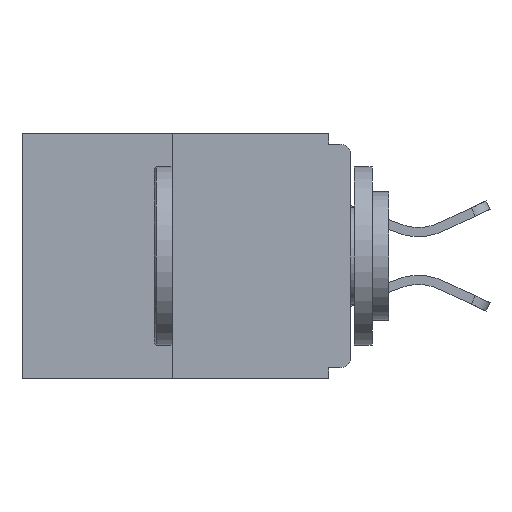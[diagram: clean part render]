
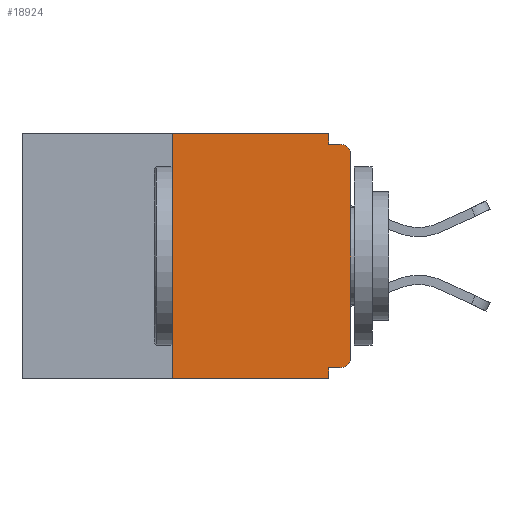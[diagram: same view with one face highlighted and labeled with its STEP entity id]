
A CAD part, left-side view. The second image highlights one B-rep face of the part: STEP entity #18924.
In plain terms, the highlighted planar face has unit normal (-1, 0, 0).
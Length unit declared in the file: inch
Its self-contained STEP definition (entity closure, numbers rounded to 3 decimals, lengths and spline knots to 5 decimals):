
#227 = EDGE_LOOP ( 'NONE', ( #14195, #5316, #4825, #1654, #13470, #17255, #25778, #17667, #17939, #3371 ) ) ;
#351 = LINE ( 'NONE', #10704, #18117 ) ;
#596 = VECTOR ( 'NONE', #18834, 39.37008 ) ;
#757 = LINE ( 'NONE', #5389, #28529 ) ;
#1392 = CARTESIAN_POINT ( 'NONE',  ( 0., 0.015, -0.015 ) ) ;
#1654 = ORIENTED_EDGE ( 'NONE', *, *, #29258, .F. ) ;
#2181 = CARTESIAN_POINT ( 'NONE',  ( 0., 0.031, -0.328 ) ) ;
#2878 = DIRECTION ( 'NONE',  ( -1., 0., 0. ) ) ;
#2971 = VERTEX_POINT ( 'NONE', #1392 ) ;
#3371 = ORIENTED_EDGE ( 'NONE', *, *, #28748, .F. ) ;
#3674 = VERTEX_POINT ( 'NONE', #2181 ) ;
#4503 = EDGE_CURVE ( 'NONE', #15290, #5673, #351, .T. ) ;
#4764 = EDGE_CURVE ( 'NONE', #24302, #2971, #10305, .T. ) ;
#4771 = CIRCLE ( 'NONE', #12991, 0.015 ) ;
#4818 = AXIS2_PLACEMENT_3D ( 'NONE', #25299, #2878, #9342 ) ;
#4825 = ORIENTED_EDGE ( 'NONE', *, *, #4503, .T. ) ;
#5074 = CARTESIAN_POINT ( 'NONE',  ( 0., 0.25, 0. ) ) ;
#5316 = ORIENTED_EDGE ( 'NONE', *, *, #17912, .F. ) ;
#5389 = CARTESIAN_POINT ( 'NONE',  ( 0., 0.031, -0.343 ) ) ;
#5435 = EDGE_CURVE ( 'NONE', #7627, #2971, #16977, .T. ) ;
#5673 = VERTEX_POINT ( 'NONE', #21308 ) ;
#7002 = CARTESIAN_POINT ( 'NONE',  ( 0., 0.031, -0.015 ) ) ;
#7541 = CARTESIAN_POINT ( 'NONE',  ( 0., 0., 0. ) ) ;
#7627 = VERTEX_POINT ( 'NONE', #18681 ) ;
#7634 = DIRECTION ( 'NONE',  ( 0., 0., -1. ) ) ;
#7929 = DIRECTION ( 'NONE',  ( 1., 0., 0. ) ) ;
#8053 = DIRECTION ( 'NONE',  ( 0., 0., -1. ) ) ;
#8394 = EDGE_CURVE ( 'NONE', #22428, #28248, #4771, .T. ) ;
#8467 = CARTESIAN_POINT ( 'NONE',  ( 0., 0.25, 0. ) ) ;
#9342 = DIRECTION ( 'NONE',  ( 0., 0., -1. ) ) ;
#10184 = EDGE_CURVE ( 'NONE', #28388, #27944, #18321, .T. ) ;
#10205 = CARTESIAN_POINT ( 'NONE',  ( 0., 0.46, 0. ) ) ;
#10285 = DIRECTION ( 'NONE',  ( 0., 0., -1. ) ) ;
#10305 = LINE ( 'NONE', #17133, #17372 ) ;
#10704 = CARTESIAN_POINT ( 'NONE',  ( 0., 0.46, -0.343 ) ) ;
#10745 = DIRECTION ( 'NONE',  ( 0., -1., 0. ) ) ;
#11199 = CARTESIAN_POINT ( 'NONE',  ( 0., 0.25, -0.343 ) ) ;
#11277 = VECTOR ( 'NONE', #14185, 39.37008 ) ;
#11306 = LINE ( 'NONE', #7541, #12731 ) ;
#11353 = CARTESIAN_POINT ( 'NONE',  ( 0., 0.031, 0. ) ) ;
#11906 = CARTESIAN_POINT ( 'NONE',  ( 0., 0.46, 0. ) ) ;
#12212 = AXIS2_PLACEMENT_3D ( 'NONE', #10205, #7929, #7634 ) ;
#12731 = VECTOR ( 'NONE', #25712, 39.37008 ) ;
#12991 = AXIS2_PLACEMENT_3D ( 'NONE', #23661, #19308, #25687 ) ;
#13470 = ORIENTED_EDGE ( 'NONE', *, *, #23976, .F. ) ;
#13720 = LINE ( 'NONE', #21492, #596 ) ;
#14185 = DIRECTION ( 'NONE',  ( 0., -1., 0. ) ) ;
#14195 = ORIENTED_EDGE ( 'NONE', *, *, #10184, .F. ) ;
#15290 = VERTEX_POINT ( 'NONE', #11199 ) ;
#15973 = CARTESIAN_POINT ( 'NONE',  ( 0., 0.015, -0.328 ) ) ;
#16977 = CIRCLE ( 'NONE', #4818, 0.015 ) ;
#17133 = CARTESIAN_POINT ( 'NONE',  ( 0., 0., -0.015 ) ) ;
#17255 = ORIENTED_EDGE ( 'NONE', *, *, #8394, .T. ) ;
#17372 = VECTOR ( 'NONE', #19623, 39.37008 ) ;
#17497 = LINE ( 'NONE', #21870, #20699 ) ;
#17667 = ORIENTED_EDGE ( 'NONE', *, *, #5435, .T. ) ;
#17912 = EDGE_CURVE ( 'NONE', #15290, #28388, #24540, .T. ) ;
#17939 = ORIENTED_EDGE ( 'NONE', *, *, #4764, .F. ) ;
#18117 = VECTOR ( 'NONE', #10745, 39.37008 ) ;
#18321 = LINE ( 'NONE', #11906, #11277 ) ;
#18681 = CARTESIAN_POINT ( 'NONE',  ( 0., 0., -0.03 ) ) ;
#18834 = DIRECTION ( 'NONE',  ( 0., 1., 0. ) ) ;
#18924 = ADVANCED_FACE ( 'NONE', ( #22720 ), #19127, .F. ) ;
#18974 = CARTESIAN_POINT ( 'NONE',  ( 0., 0., -0.313 ) ) ;
#19127 = PLANE ( 'NONE',  #12212 ) ;
#19308 = DIRECTION ( 'NONE',  ( -1., 0., 0. ) ) ;
#19623 = DIRECTION ( 'NONE',  ( 0., -1., 0. ) ) ;
#20139 = EDGE_CURVE ( 'NONE', #28248, #7627, #11306, .T. ) ;
#20699 = VECTOR ( 'NONE', #10285, 39.37008 ) ;
#20928 = DIRECTION ( 'NONE',  ( 0., 0., 1. ) ) ;
#21308 = CARTESIAN_POINT ( 'NONE',  ( 0., 0.031, -0.343 ) ) ;
#21492 = CARTESIAN_POINT ( 'NONE',  ( 0., 0., -0.328 ) ) ;
#21870 = CARTESIAN_POINT ( 'NONE',  ( 0., 0.031, 0. ) ) ;
#22428 = VERTEX_POINT ( 'NONE', #15973 ) ;
#22720 = FACE_OUTER_BOUND ( 'NONE', #227, .T. ) ;
#23661 = CARTESIAN_POINT ( 'NONE',  ( 0., 0.015, -0.313 ) ) ;
#23976 = EDGE_CURVE ( 'NONE', #22428, #3674, #13720, .T. ) ;
#24302 = VERTEX_POINT ( 'NONE', #7002 ) ;
#24540 = LINE ( 'NONE', #5074, #27790 ) ;
#25299 = CARTESIAN_POINT ( 'NONE',  ( 0., 0.015, -0.03 ) ) ;
#25687 = DIRECTION ( 'NONE',  ( 0., 0., -1. ) ) ;
#25712 = DIRECTION ( 'NONE',  ( 0., 0., 1. ) ) ;
#25778 = ORIENTED_EDGE ( 'NONE', *, *, #20139, .T. ) ;
#27790 = VECTOR ( 'NONE', #20928, 39.37008 ) ;
#27944 = VERTEX_POINT ( 'NONE', #11353 ) ;
#28248 = VERTEX_POINT ( 'NONE', #18974 ) ;
#28388 = VERTEX_POINT ( 'NONE', #8467 ) ;
#28529 = VECTOR ( 'NONE', #8053, 39.37008 ) ;
#28748 = EDGE_CURVE ( 'NONE', #27944, #24302, #17497, .T. ) ;
#29258 = EDGE_CURVE ( 'NONE', #3674, #5673, #757, .T. ) ;
